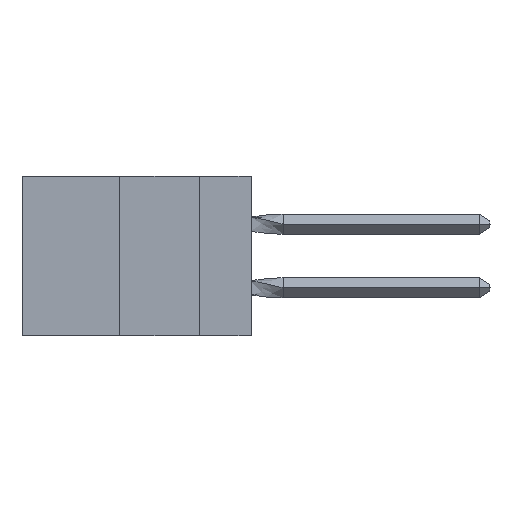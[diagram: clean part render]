
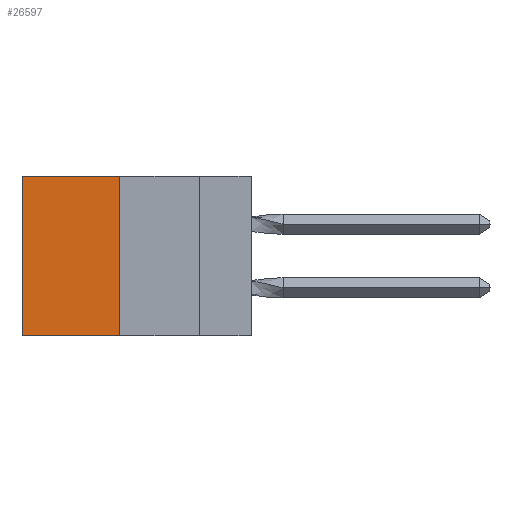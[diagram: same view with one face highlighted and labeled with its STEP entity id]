
A CAD part, left-side view. The second image highlights one B-rep face of the part: STEP entity #26597.
In plain terms, the highlighted planar face has unit normal (-1, 0, 0).
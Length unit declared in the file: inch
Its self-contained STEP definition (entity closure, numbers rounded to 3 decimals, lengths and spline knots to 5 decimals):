
#874 = VECTOR ( 'NONE', #30756, 39.37008 ) ;
#922 = CARTESIAN_POINT ( 'NONE',  ( 0.305, 0.413, -0.5 ) ) ;
#1724 = DIRECTION ( 'NONE',  ( 0., 1., 0. ) ) ;
#2384 = EDGE_CURVE ( 'NONE', #16036, #9344, #16242, .T. ) ;
#3459 = DIRECTION ( 'NONE',  ( 0., 1., 0. ) ) ;
#4884 = CARTESIAN_POINT ( 'NONE',  ( 0.305, 0.413, -0.5 ) ) ;
#5009 = LINE ( 'NONE', #922, #29654 ) ;
#5958 = EDGE_CURVE ( 'NONE', #16036, #25503, #18824, .T. ) ;
#8460 = PLANE ( 'NONE',  #13721 ) ;
#9344 = VERTEX_POINT ( 'NONE', #4884 ) ;
#12601 = FACE_OUTER_BOUND ( 'NONE', #30339, .T. ) ;
#13213 = VECTOR ( 'NONE', #1724, 39.37008 ) ;
#13480 = CARTESIAN_POINT ( 'NONE',  ( 0.305, 0.72, -0.5 ) ) ;
#13721 = AXIS2_PLACEMENT_3D ( 'NONE', #27596, #25392, #18155 ) ;
#14041 = ORIENTED_EDGE ( 'NONE', *, *, #28559, .F. ) ;
#14192 = DIRECTION ( 'NONE',  ( 0., 0., -1. ) ) ;
#15057 = ORIENTED_EDGE ( 'NONE', *, *, #2384, .F. ) ;
#16036 = VERTEX_POINT ( 'NONE', #18488 ) ;
#16242 = LINE ( 'NONE', #18442, #874 ) ;
#18155 = DIRECTION ( 'NONE',  ( 0., 0., -1. ) ) ;
#18257 = CARTESIAN_POINT ( 'NONE',  ( 0.305, 0.413, 0. ) ) ;
#18442 = CARTESIAN_POINT ( 'NONE',  ( 0.305, 0.413, -0.5 ) ) ;
#18488 = CARTESIAN_POINT ( 'NONE',  ( 0.305, 0.413, 0. ) ) ;
#18824 = LINE ( 'NONE', #18257, #13213 ) ;
#20951 = ORIENTED_EDGE ( 'NONE', *, *, #26069, .T. ) ;
#22539 = VERTEX_POINT ( 'NONE', #13480 ) ;
#22708 = LINE ( 'NONE', #30336, #29836 ) ;
#25392 = DIRECTION ( 'NONE',  ( 1., 0., 0. ) ) ;
#25503 = VERTEX_POINT ( 'NONE', #30866 ) ;
#26069 = EDGE_CURVE ( 'NONE', #25503, #22539, #22708, .T. ) ;
#26597 = ADVANCED_FACE ( 'NONE', ( #12601 ), #8460, .F. ) ;
#27596 = CARTESIAN_POINT ( 'NONE',  ( 0.305, 0.413, -0.5 ) ) ;
#28559 = EDGE_CURVE ( 'NONE', #9344, #22539, #5009, .T. ) ;
#29654 = VECTOR ( 'NONE', #3459, 39.37008 ) ;
#29836 = VECTOR ( 'NONE', #14192, 39.37008 ) ;
#30336 = CARTESIAN_POINT ( 'NONE',  ( 0.305, 0.72, -0.5 ) ) ;
#30339 = EDGE_LOOP ( 'NONE', ( #20951, #14041, #15057, #30704 ) ) ;
#30704 = ORIENTED_EDGE ( 'NONE', *, *, #5958, .T. ) ;
#30756 = DIRECTION ( 'NONE',  ( 0., 0., -1. ) ) ;
#30866 = CARTESIAN_POINT ( 'NONE',  ( 0.305, 0.72, 0. ) ) ;
